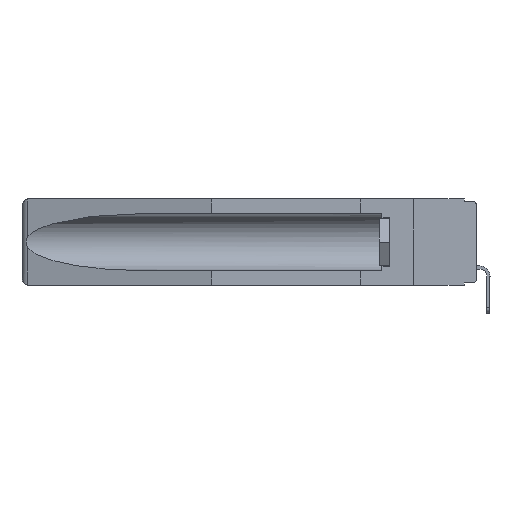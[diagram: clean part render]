
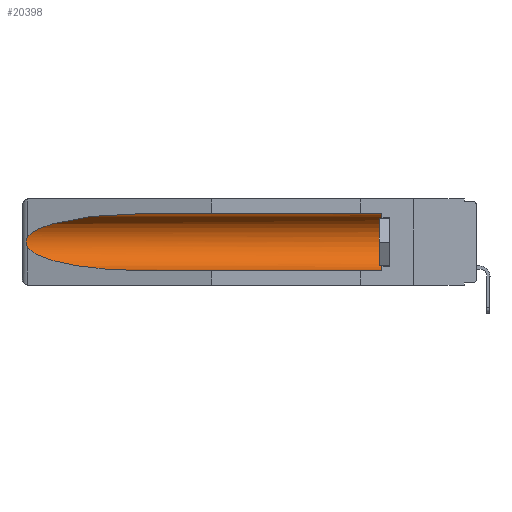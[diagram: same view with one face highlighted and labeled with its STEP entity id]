
A CAD part, left-side view. The second image highlights one B-rep face of the part: STEP entity #20398.
In plain terms, the highlighted cylindrical face has radius 2.857 mm (diameter 5.715 mm), a partial arc.
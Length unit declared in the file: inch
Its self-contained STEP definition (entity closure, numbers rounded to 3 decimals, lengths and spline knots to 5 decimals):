
#1713 = VERTEX_POINT ( 'NONE', #7732 ) ;
#1728 = CARTESIAN_POINT ( 'NONE',  ( 0.155, 1.07973, -0.284 ) ) ;
#2422 = CARTESIAN_POINT ( 'NONE',  ( 0.25451, 1.48313, -0.09465 ) ) ;
#2648 = DIRECTION ( 'NONE',  ( 0., 0., 1. ) ) ;
#2703 = CARTESIAN_POINT ( 'NONE',  ( 0.26537, 1.52718, -0.14972 ) ) ;
#2788 = AXIS2_PLACEMENT_3D ( 'NONE', #11386, #19607, #11248 ) ;
#3118 = CARTESIAN_POINT ( 'NONE',  ( 0.26597, 1.52961, -0.15275 ) ) ;
#3712 = VECTOR ( 'NONE', #8632, 39.37008 ) ;
#4305 = ORIENTED_EDGE ( 'NONE', *, *, #13095, .T. ) ;
#4721 = CARTESIAN_POINT ( 'NONE',  ( 0.155, -0.30754, -0.284 ) ) ;
#4734 = CARTESIAN_POINT ( 'NONE',  ( 0.155, -0.30754, -0.1715 ) ) ;
#5222 =( BOUNDED_CURVE ( )  B_SPLINE_CURVE ( 3, ( #26126, #19171, #2422, #15543 ),
 .UNSPECIFIED., .F., .T. ) 
 B_SPLINE_CURVE_WITH_KNOTS ( ( 4, 4 ),
 ( 4.71239, 6.08839 ),
 .UNSPECIFIED. ) 
 CURVE ( )  GEOMETRIC_REPRESENTATION_ITEM ( )  RATIONAL_B_SPLINE_CURVE ( ( 1., 0.848, 0.848, 1. ) ) 
 REPRESENTATION_ITEM ( '' )  );
#5692 = EDGE_LOOP ( 'NONE', ( #4305, #7783, #22808, #7147, #24203, #13047 ) ) ;
#5917 = CARTESIAN_POINT ( 'NONE',  ( 0.26537, 1.52718, -0.19328 ) ) ;
#6198 = CARTESIAN_POINT ( 'NONE',  ( 0.21114, 1.30732, -0.284 ) ) ;
#6755 = VERTEX_POINT ( 'NONE', #2703 ) ;
#7147 = ORIENTED_EDGE ( 'NONE', *, *, #25515, .F. ) ;
#7586 = CARTESIAN_POINT ( 'NONE',  ( 0.2675, 1.53308, -0.16763 ) ) ;
#7722 = CARTESIAN_POINT ( 'NONE',  ( 0.2673, 1.53269, -0.17917 ) ) ;
#7732 = CARTESIAN_POINT ( 'NONE',  ( 0.155, 0.126, -0.284 ) ) ;
#7783 = ORIENTED_EDGE ( 'NONE', *, *, #19701, .T. ) ;
#8147 = VECTOR ( 'NONE', #17851, 39.37008 ) ;
#8511 = FACE_OUTER_BOUND ( 'NONE', #5692, .T. ) ;
#8632 = DIRECTION ( 'NONE',  ( 0., 1., 0. ) ) ;
#8787 = VERTEX_POINT ( 'NONE', #9071 ) ;
#9071 = CARTESIAN_POINT ( 'NONE',  ( 0.155, 0.126, -0.059 ) ) ;
#9134 =( BOUNDED_CURVE ( )  B_SPLINE_CURVE ( 3, ( #5917, #22932, #6198, #1728 ),
 .UNSPECIFIED., .F., .T. ) 
 B_SPLINE_CURVE_WITH_KNOTS ( ( 4, 4 ),
 ( 0.1948, 1.5708 ),
 .UNSPECIFIED. ) 
 CURVE ( )  GEOMETRIC_REPRESENTATION_ITEM ( )  RATIONAL_B_SPLINE_CURVE ( ( 1., 0.848, 0.848, 1. ) ) 
 REPRESENTATION_ITEM ( '' )  );
#9489 = CARTESIAN_POINT ( 'NONE',  ( 0.26537, 1.52718, -0.19328 ) ) ;
#10611 = EDGE_CURVE ( 'NONE', #20543, #20469, #9134, .T. ) ;
#10757 = DIRECTION ( 'NONE',  ( 0., 1., 0. ) ) ;
#11248 = DIRECTION ( 'NONE',  ( 0., 0., 1. ) ) ;
#11386 = CARTESIAN_POINT ( 'NONE',  ( 0.155, 0.126, -0.1715 ) ) ;
#11825 = VERTEX_POINT ( 'NONE', #23483 ) ;
#12155 = B_SPLINE_CURVE_WITH_KNOTS ( 'NONE', 3,
 ( #18334, #3118, #14151, #26824, #7586, #26412, #7722, #16108, #22105, #20552 ),
 .UNSPECIFIED., .F., .F.,
 ( 4, 2, 2, 2, 4 ),
 ( 0., 0.00029, 0.00058, 0.00087, 0.00117 ),
 .UNSPECIFIED. ) ;
#12598 = CIRCLE ( 'NONE', #2788, 0.1125 ) ;
#13047 = ORIENTED_EDGE ( 'NONE', *, *, #26350, .T. ) ;
#13095 = EDGE_CURVE ( 'NONE', #11825, #6755, #5222, .T. ) ;
#14151 = CARTESIAN_POINT ( 'NONE',  ( 0.26654, 1.53092, -0.15636 ) ) ;
#15543 = CARTESIAN_POINT ( 'NONE',  ( 0.26537, 1.52718, -0.14972 ) ) ;
#16108 = CARTESIAN_POINT ( 'NONE',  ( 0.26655, 1.53094, -0.18657 ) ) ;
#17021 = LINE ( 'NONE', #21729, #3712 ) ;
#17036 = CYLINDRICAL_SURFACE ( 'NONE', #24376, 0.1125 ) ;
#17851 = DIRECTION ( 'NONE',  ( 0., 1., 0. ) ) ;
#18334 = CARTESIAN_POINT ( 'NONE',  ( 0.26537, 1.52718, -0.14972 ) ) ;
#19171 = CARTESIAN_POINT ( 'NONE',  ( 0.21114, 1.30732, -0.059 ) ) ;
#19607 = DIRECTION ( 'NONE',  ( 0., -1., 0. ) ) ;
#19701 = EDGE_CURVE ( 'NONE', #6755, #20543, #12155, .T. ) ;
#20398 = ADVANCED_FACE ( 'NONE', ( #8511 ), #17036, .F. ) ;
#20469 = VERTEX_POINT ( 'NONE', #26495 ) ;
#20543 = VERTEX_POINT ( 'NONE', #9489 ) ;
#20552 = CARTESIAN_POINT ( 'NONE',  ( 0.26537, 1.52718, -0.19328 ) ) ;
#21729 = CARTESIAN_POINT ( 'NONE',  ( 0.155, -0.30754, -0.059 ) ) ;
#22105 = CARTESIAN_POINT ( 'NONE',  ( 0.26597, 1.5296, -0.19026 ) ) ;
#22808 = ORIENTED_EDGE ( 'NONE', *, *, #10611, .T. ) ;
#22932 = CARTESIAN_POINT ( 'NONE',  ( 0.25451, 1.48313, -0.24835 ) ) ;
#23483 = CARTESIAN_POINT ( 'NONE',  ( 0.155, 1.07973, -0.059 ) ) ;
#23984 = LINE ( 'NONE', #4721, #8147 ) ;
#24203 = ORIENTED_EDGE ( 'NONE', *, *, #25755, .T. ) ;
#24376 = AXIS2_PLACEMENT_3D ( 'NONE', #4734, #10757, #2648 ) ;
#25515 = EDGE_CURVE ( 'NONE', #1713, #20469, #23984, .T. ) ;
#25755 = EDGE_CURVE ( 'NONE', #1713, #8787, #12598, .T. ) ;
#26126 = CARTESIAN_POINT ( 'NONE',  ( 0.155, 1.07973, -0.059 ) ) ;
#26350 = EDGE_CURVE ( 'NONE', #8787, #11825, #17021, .T. ) ;
#26412 = CARTESIAN_POINT ( 'NONE',  ( 0.2675, 1.53308, -0.17534 ) ) ;
#26495 = CARTESIAN_POINT ( 'NONE',  ( 0.155, 1.07973, -0.284 ) ) ;
#26824 = CARTESIAN_POINT ( 'NONE',  ( 0.2673, 1.5327, -0.16383 ) ) ;
